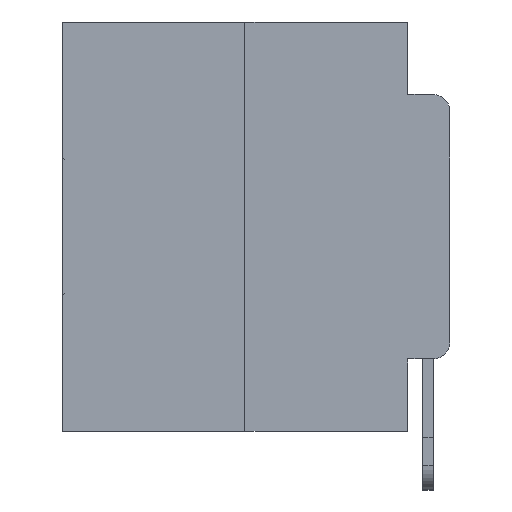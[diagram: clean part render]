
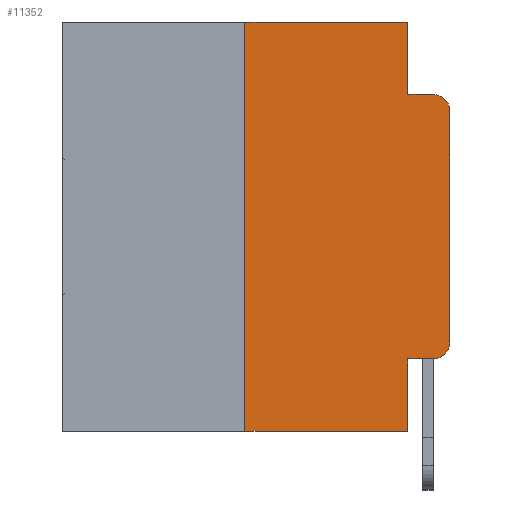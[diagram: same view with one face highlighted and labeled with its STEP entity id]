
A CAD part, left-side view. The second image highlights one B-rep face of the part: STEP entity #11352.
In plain terms, the highlighted planar face has unit normal (-1, 0, 0).
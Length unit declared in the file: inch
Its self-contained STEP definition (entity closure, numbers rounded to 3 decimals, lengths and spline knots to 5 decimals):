
#118 = VERTEX_POINT ( 'NONE', #10023 ) ;
#505 = DIRECTION ( 'NONE',  ( 0., -1., 0. ) ) ;
#579 = CARTESIAN_POINT ( 'NONE',  ( 0., 0.02, -0.3915 ) ) ;
#652 = DIRECTION ( 'NONE',  ( 0., 0., 1. ) ) ;
#791 = LINE ( 'NONE', #20730, #24451 ) ;
#2249 = ORIENTED_EDGE ( 'NONE', *, *, #21657, .T. ) ;
#3042 = DIRECTION ( 'NONE',  ( 0., 0., -1. ) ) ;
#3339 = CARTESIAN_POINT ( 'NONE',  ( 0., 0., -0.3915 ) ) ;
#3547 = ORIENTED_EDGE ( 'NONE', *, *, #9457, .F. ) ;
#4567 = LINE ( 'NONE', #19827, #27868 ) ;
#4862 = EDGE_CURVE ( 'NONE', #118, #26227, #23079, .T. ) ;
#4961 = CARTESIAN_POINT ( 'NONE',  ( 0., 0.051, -0.0885 ) ) ;
#5083 = EDGE_CURVE ( 'NONE', #118, #22602, #4567, .T. ) ;
#6171 = DIRECTION ( 'NONE',  ( 0., -1., 0. ) ) ;
#6779 = DIRECTION ( 'NONE',  ( 0., 0., -1. ) ) ;
#6874 = VERTEX_POINT ( 'NONE', #17885 ) ;
#7344 = LINE ( 'NONE', #8109, #8061 ) ;
#7661 = VECTOR ( 'NONE', #6779, 39.37008 ) ;
#8061 = VECTOR ( 'NONE', #21738, 39.37008 ) ;
#8109 = CARTESIAN_POINT ( 'NONE',  ( 0., 0.051, -0.0885 ) ) ;
#8414 = VECTOR ( 'NONE', #652, 39.37008 ) ;
#8635 = CIRCLE ( 'NONE', #15025, 0.02 ) ;
#9369 = PLANE ( 'NONE',  #23999 ) ;
#9457 = EDGE_CURVE ( 'NONE', #13924, #23329, #791, .T. ) ;
#9831 = CARTESIAN_POINT ( 'NONE',  ( 0., 0.051, -0.4115 ) ) ;
#9853 = ORIENTED_EDGE ( 'NONE', *, *, #18631, .T. ) ;
#10023 = CARTESIAN_POINT ( 'NONE',  ( 0., 0.25, -0.5 ) ) ;
#10755 = DIRECTION ( 'NONE',  ( -1., 0., 0. ) ) ;
#11008 = EDGE_CURVE ( 'NONE', #23329, #11187, #7344, .T. ) ;
#11049 = LINE ( 'NONE', #12150, #22405 ) ;
#11187 = VERTEX_POINT ( 'NONE', #20157 ) ;
#11352 = ADVANCED_FACE ( 'NONE', ( #27420 ), #9369, .F. ) ;
#12150 = CARTESIAN_POINT ( 'NONE',  ( 0., 0.473, 0. ) ) ;
#13056 = LINE ( 'NONE', #22652, #7661 ) ;
#13142 = EDGE_CURVE ( 'NONE', #6874, #21208, #8635, .T. ) ;
#13200 = CARTESIAN_POINT ( 'NONE',  ( 0., 0.051, 0. ) ) ;
#13417 = AXIS2_PLACEMENT_3D ( 'NONE', #24297, #10755, #26514 ) ;
#13669 = ORIENTED_EDGE ( 'NONE', *, *, #26652, .F. ) ;
#13924 = VERTEX_POINT ( 'NONE', #13200 ) ;
#13968 = CIRCLE ( 'NONE', #13417, 0.02 ) ;
#14009 = DIRECTION ( 'NONE',  ( 0., 0., -1. ) ) ;
#14469 = DIRECTION ( 'NONE',  ( 0., -1., 0. ) ) ;
#15025 = AXIS2_PLACEMENT_3D ( 'NONE', #579, #16815, #3042 ) ;
#16265 = VECTOR ( 'NONE', #505, 39.37008 ) ;
#16430 = VECTOR ( 'NONE', #27833, 39.37008 ) ;
#16519 = ORIENTED_EDGE ( 'NONE', *, *, #13142, .T. ) ;
#16636 = CARTESIAN_POINT ( 'NONE',  ( 0., 0., -0.1085 ) ) ;
#16784 = CARTESIAN_POINT ( 'NONE',  ( 0., 0., 0. ) ) ;
#16815 = DIRECTION ( 'NONE',  ( -1., 0., 0. ) ) ;
#16985 = LINE ( 'NONE', #9831, #16265 ) ;
#17885 = CARTESIAN_POINT ( 'NONE',  ( 0., 0.02, -0.4115 ) ) ;
#18631 = EDGE_CURVE ( 'NONE', #25390, #11187, #13968, .T. ) ;
#19298 = ORIENTED_EDGE ( 'NONE', *, *, #29401, .F. ) ;
#19651 = ORIENTED_EDGE ( 'NONE', *, *, #11008, .F. ) ;
#19827 = CARTESIAN_POINT ( 'NONE',  ( 0., 0.473, -0.5 ) ) ;
#20157 = CARTESIAN_POINT ( 'NONE',  ( 0., 0.02, -0.0885 ) ) ;
#20359 = CARTESIAN_POINT ( 'NONE',  ( 0., 0.051, -0.5 ) ) ;
#20730 = CARTESIAN_POINT ( 'NONE',  ( 0., 0.051, 0. ) ) ;
#21084 = ORIENTED_EDGE ( 'NONE', *, *, #22221, .T. ) ;
#21207 = CARTESIAN_POINT ( 'NONE',  ( 0., 0.25, 0. ) ) ;
#21208 = VERTEX_POINT ( 'NONE', #3339 ) ;
#21657 = EDGE_CURVE ( 'NONE', #21208, #25390, #26433, .T. ) ;
#21738 = DIRECTION ( 'NONE',  ( 0., -1., 0. ) ) ;
#22221 = EDGE_CURVE ( 'NONE', #28853, #6874, #16985, .T. ) ;
#22258 = CARTESIAN_POINT ( 'NONE',  ( 0., 0.051, -0.4115 ) ) ;
#22405 = VECTOR ( 'NONE', #14469, 39.37008 ) ;
#22602 = VERTEX_POINT ( 'NONE', #20359 ) ;
#22652 = CARTESIAN_POINT ( 'NONE',  ( 0., 0.051, 0. ) ) ;
#22810 = ORIENTED_EDGE ( 'NONE', *, *, #5083, .T. ) ;
#22967 = DIRECTION ( 'NONE',  ( 0., 0., -1. ) ) ;
#23079 = LINE ( 'NONE', #21207, #16430 ) ;
#23329 = VERTEX_POINT ( 'NONE', #4961 ) ;
#23999 = AXIS2_PLACEMENT_3D ( 'NONE', #25212, #27389, #14009 ) ;
#24297 = CARTESIAN_POINT ( 'NONE',  ( 0., 0.02, -0.1085 ) ) ;
#24451 = VECTOR ( 'NONE', #22967, 39.37008 ) ;
#25212 = CARTESIAN_POINT ( 'NONE',  ( 0., 0.473, 0. ) ) ;
#25390 = VERTEX_POINT ( 'NONE', #16636 ) ;
#26226 = EDGE_LOOP ( 'NONE', ( #2249, #9853, #19651, #3547, #19298, #27284, #22810, #13669, #21084, #16519 ) ) ;
#26227 = VERTEX_POINT ( 'NONE', #27662 ) ;
#26433 = LINE ( 'NONE', #16784, #8414 ) ;
#26514 = DIRECTION ( 'NONE',  ( 0., 0., -1. ) ) ;
#26652 = EDGE_CURVE ( 'NONE', #28853, #22602, #13056, .T. ) ;
#27284 = ORIENTED_EDGE ( 'NONE', *, *, #4862, .F. ) ;
#27389 = DIRECTION ( 'NONE',  ( 1., 0., 0. ) ) ;
#27420 = FACE_OUTER_BOUND ( 'NONE', #26226, .T. ) ;
#27662 = CARTESIAN_POINT ( 'NONE',  ( 0., 0.25, 0. ) ) ;
#27833 = DIRECTION ( 'NONE',  ( 0., 0., 1. ) ) ;
#27868 = VECTOR ( 'NONE', #6171, 39.37008 ) ;
#28853 = VERTEX_POINT ( 'NONE', #22258 ) ;
#29401 = EDGE_CURVE ( 'NONE', #26227, #13924, #11049, .T. ) ;
